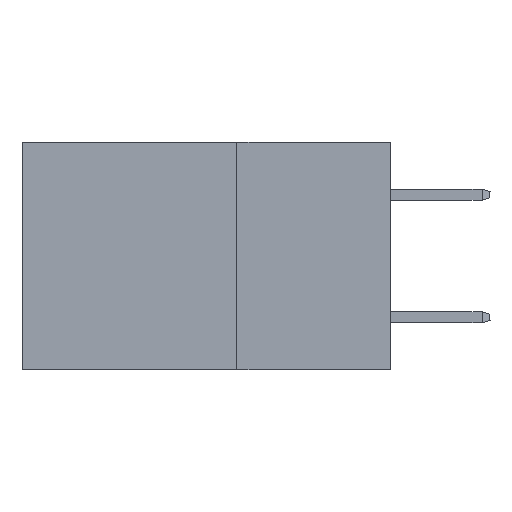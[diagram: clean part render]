
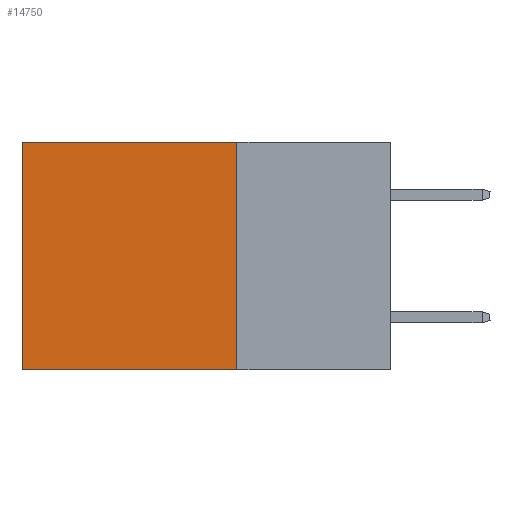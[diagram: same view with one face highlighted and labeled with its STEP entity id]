
A CAD part, left-side view. The second image highlights one B-rep face of the part: STEP entity #14750.
In plain terms, the highlighted planar face has unit normal (-1, 0, 0).
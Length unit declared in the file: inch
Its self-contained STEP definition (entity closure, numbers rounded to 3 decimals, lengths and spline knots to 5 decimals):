
#98 = VERTEX_POINT ( 'NONE', #12541 ) ;
#389 = LINE ( 'NONE', #18917, #17436 ) ;
#2449 = VECTOR ( 'NONE', #11427, 39.37008 ) ;
#2680 = EDGE_LOOP ( 'NONE', ( #17368, #21645, #15551, #24389 ) ) ;
#3955 = LINE ( 'NONE', #28448, #9365 ) ;
#4112 = CARTESIAN_POINT ( 'NONE',  ( 0.2875, 0.25, 0. ) ) ;
#4467 = DIRECTION ( 'NONE',  ( 0., 1., 0. ) ) ;
#4552 = VERTEX_POINT ( 'NONE', #14632 ) ;
#6439 = DIRECTION ( 'NONE',  ( 1., 0., 0. ) ) ;
#7975 = VERTEX_POINT ( 'NONE', #19561 ) ;
#8656 = VECTOR ( 'NONE', #4467, 39.37008 ) ;
#9365 = VECTOR ( 'NONE', #10085, 39.37008 ) ;
#9735 = AXIS2_PLACEMENT_3D ( 'NONE', #4112, #6439, #22599 ) ;
#10085 = DIRECTION ( 'NONE',  ( 0., 0., -1. ) ) ;
#10738 = EDGE_CURVE ( 'NONE', #25033, #4552, #3955, .T. ) ;
#11427 = DIRECTION ( 'NONE',  ( 0., 1., 0. ) ) ;
#12541 = CARTESIAN_POINT ( 'NONE',  ( 0.2875, 0.6, -0.37 ) ) ;
#13831 = EDGE_CURVE ( 'NONE', #7975, #98, #389, .T. ) ;
#14632 = CARTESIAN_POINT ( 'NONE',  ( 0.2875, 0.25, -0.37 ) ) ;
#14750 = ADVANCED_FACE ( 'NONE', ( #16645 ), #17965, .F. ) ;
#14845 = LINE ( 'NONE', #29667, #8656 ) ;
#15551 = ORIENTED_EDGE ( 'NONE', *, *, #10738, .F. ) ;
#15742 = CARTESIAN_POINT ( 'NONE',  ( 0.2875, 0.25, 0. ) ) ;
#15984 = EDGE_CURVE ( 'NONE', #4552, #98, #25550, .T. ) ;
#16645 = FACE_OUTER_BOUND ( 'NONE', #2680, .T. ) ;
#17368 = ORIENTED_EDGE ( 'NONE', *, *, #13831, .T. ) ;
#17436 = VECTOR ( 'NONE', #21225, 39.37008 ) ;
#17965 = PLANE ( 'NONE',  #9735 ) ;
#18917 = CARTESIAN_POINT ( 'NONE',  ( 0.2875, 0.6, 0. ) ) ;
#19561 = CARTESIAN_POINT ( 'NONE',  ( 0.2875, 0.6, 0. ) ) ;
#21225 = DIRECTION ( 'NONE',  ( 0., 0., -1. ) ) ;
#21645 = ORIENTED_EDGE ( 'NONE', *, *, #15984, .F. ) ;
#22599 = DIRECTION ( 'NONE',  ( 0., 0., -1. ) ) ;
#24389 = ORIENTED_EDGE ( 'NONE', *, *, #28505, .T. ) ;
#25033 = VERTEX_POINT ( 'NONE', #15742 ) ;
#25212 = CARTESIAN_POINT ( 'NONE',  ( 0.2875, 0.25, -0.37 ) ) ;
#25550 = LINE ( 'NONE', #25212, #2449 ) ;
#28448 = CARTESIAN_POINT ( 'NONE',  ( 0.2875, 0.25, 0. ) ) ;
#28505 = EDGE_CURVE ( 'NONE', #25033, #7975, #14845, .T. ) ;
#29667 = CARTESIAN_POINT ( 'NONE',  ( 0.2875, 0.25, 0. ) ) ;
